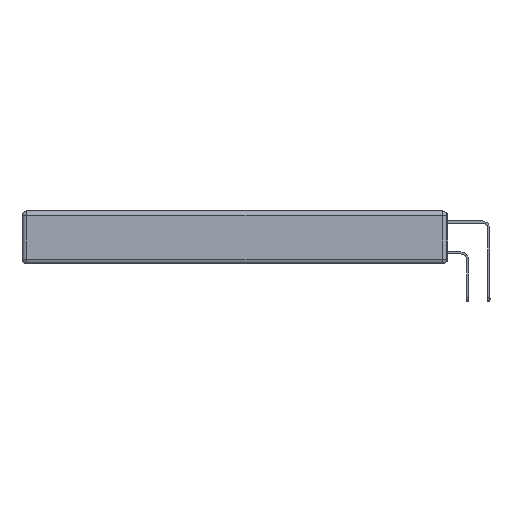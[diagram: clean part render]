
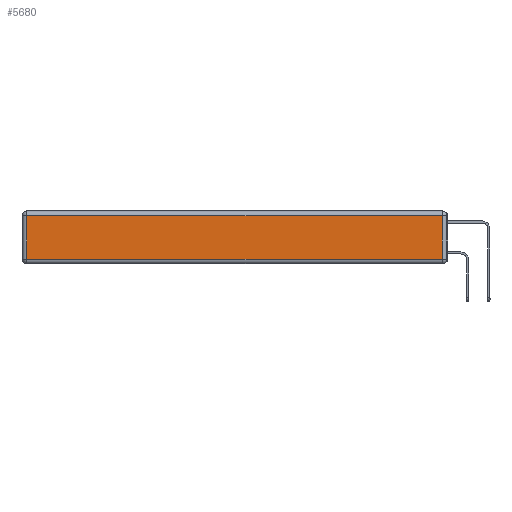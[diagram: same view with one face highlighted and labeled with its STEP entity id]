
A CAD part, left-side view. The second image highlights one B-rep face of the part: STEP entity #5680.
In plain terms, the highlighted planar face has unit normal (-1, 0, 0).
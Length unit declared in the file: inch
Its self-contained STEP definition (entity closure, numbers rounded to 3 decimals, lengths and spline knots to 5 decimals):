
#85 = VECTOR ( 'NONE', #16037, 39.37008 ) ;
#354 = AXIS2_PLACEMENT_3D ( 'NONE', #8740, #20918, #9189 ) ;
#1510 = VERTEX_POINT ( 'NONE', #18582 ) ;
#2068 = PLANE ( 'NONE',  #354 ) ;
#2184 = EDGE_CURVE ( 'NONE', #1510, #5591, #21174, .T. ) ;
#2313 = ORIENTED_EDGE ( 'NONE', *, *, #4834, .T. ) ;
#2657 = CARTESIAN_POINT ( 'NONE',  ( 0., 0.03, -0.343 ) ) ;
#3818 = CARTESIAN_POINT ( 'NONE',  ( 0., 0.03, -0.03 ) ) ;
#4026 = CARTESIAN_POINT ( 'NONE',  ( 0., 2.72, -0.343 ) ) ;
#4834 = EDGE_CURVE ( 'NONE', #19270, #1510, #14276, .T. ) ;
#5591 = VERTEX_POINT ( 'NONE', #3818 ) ;
#5655 = LINE ( 'NONE', #4026, #15564 ) ;
#5680 = ADVANCED_FACE ( 'NONE', ( #10383 ), #2068, .T. ) ;
#6256 = EDGE_CURVE ( 'NONE', #16733, #19270, #5655, .T. ) ;
#6581 = CARTESIAN_POINT ( 'NONE',  ( 0., 2.72, -0.03 ) ) ;
#6909 = EDGE_LOOP ( 'NONE', ( #2313, #19588, #17402, #7315 ) ) ;
#7315 = ORIENTED_EDGE ( 'NONE', *, *, #6256, .T. ) ;
#8740 = CARTESIAN_POINT ( 'NONE',  ( 0., 0., -0.343 ) ) ;
#9189 = DIRECTION ( 'NONE',  ( 0., 0., 1. ) ) ;
#9758 = DIRECTION ( 'NONE',  ( 0., 0., 1. ) ) ;
#10383 = FACE_OUTER_BOUND ( 'NONE', #6909, .T. ) ;
#10611 = LINE ( 'NONE', #12137, #19347 ) ;
#10678 = DIRECTION ( 'NONE',  ( 0., 0., -1. ) ) ;
#12137 = CARTESIAN_POINT ( 'NONE',  ( 0., 2.75, -0.03 ) ) ;
#13279 = VECTOR ( 'NONE', #9758, 39.37008 ) ;
#14276 = LINE ( 'NONE', #14606, #85 ) ;
#14606 = CARTESIAN_POINT ( 'NONE',  ( 0., 0., -0.313 ) ) ;
#15564 = VECTOR ( 'NONE', #10678, 39.37008 ) ;
#15954 = CARTESIAN_POINT ( 'NONE',  ( 0., 2.72, -0.313 ) ) ;
#16037 = DIRECTION ( 'NONE',  ( 0., -1., 0. ) ) ;
#16733 = VERTEX_POINT ( 'NONE', #6581 ) ;
#16976 = EDGE_CURVE ( 'NONE', #5591, #16733, #10611, .T. ) ;
#17316 = DIRECTION ( 'NONE',  ( 0., 1., 0. ) ) ;
#17402 = ORIENTED_EDGE ( 'NONE', *, *, #16976, .T. ) ;
#18582 = CARTESIAN_POINT ( 'NONE',  ( 0., 0.03, -0.313 ) ) ;
#19270 = VERTEX_POINT ( 'NONE', #15954 ) ;
#19347 = VECTOR ( 'NONE', #17316, 39.37008 ) ;
#19588 = ORIENTED_EDGE ( 'NONE', *, *, #2184, .T. ) ;
#20918 = DIRECTION ( 'NONE',  ( -1., 0., 0. ) ) ;
#21174 = LINE ( 'NONE', #2657, #13279 ) ;
